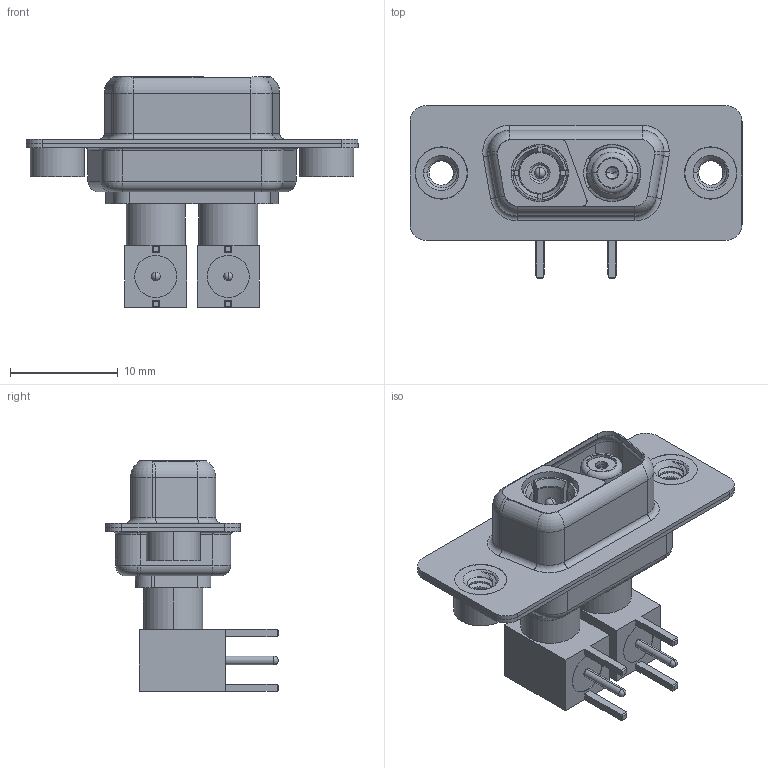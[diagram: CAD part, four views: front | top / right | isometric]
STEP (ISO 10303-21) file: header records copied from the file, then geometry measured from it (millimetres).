
FILE_DESCRIPTION (( 'STEP AP203' ), '1' );
FILE_NAME ('630-2WK2240-7T2.STEP', '2022-05-26T23:45:32', ( '' ), ( '' ), 'SwSTEP 2.0', 'SolidWorks 2020', '' );
FILE_SCHEMA (( 'CONFIG_CONTROL_DESIGN' ));
Length unit declared in the file: millimetre
Products named in the file (17): Co-Ax Plug Assy_RA; 630Combo Shell Front_09 Contacts; Insulator RA Pin; 630-2WK2240-7T2; RA Back Shell; Insulator Socket; Locking Collar; Co-Ax Plug_RA PC Tail; Co-Ax Jack_RA PC Tail; Co-Ax Jack Assy_RA; Insulator Pin_Straight PC Tail; 630Combo Shell Rear_09 Contacts; 630Combo Housing_2WK2; Pin_RA; Socket_RA; Insulator Socket 2; 630Combo Threaded Rivet_2
Assembly tree (20 placements, depth 3):
  630-2WK2240-7T2
    630Combo Housing_2WK2
    630Combo Shell Front_09 Contacts
    630Combo Shell Rear_09 Contacts
    630Combo Threaded Rivet_2  x2
    Co-Ax Plug Assy_RA
      Co-Ax Plug_RA PC Tail
      Insulator Pin_Straight PC Tail
      Pin_RA
      Locking Collar
      RA Back Shell
      Insulator RA Pin
    Co-Ax Jack Assy_RA
      Co-Ax Jack_RA PC Tail
      Insulator Socket
      Insulator Socket 2
      Locking Collar
      Socket_RA
      RA Back Shell
      Insulator RA Pin
Bounding box: 30.8 x 16 x 21.41 mm (x, y, z)
Volume: 2012.2 mm3; surface area: 5567.9 mm2
Topology: 18 solids, 18 shells, 600 faces, 1434 edges, 893 vertices
Faces by surface type: cylinder 270, plane 191, torus 69, cone 56, bspline 8, sphere 6
Entity records: 18421 total; most frequent: CARTESIAN_POINT 4429, DIRECTION 2733, ORIENTED_EDGE 2400, EDGE_CURVE 1200, AXIS2_PLACEMENT_3D 1113, VERTEX_POINT 756, CIRCLE 582, EDGE_LOOP 580
